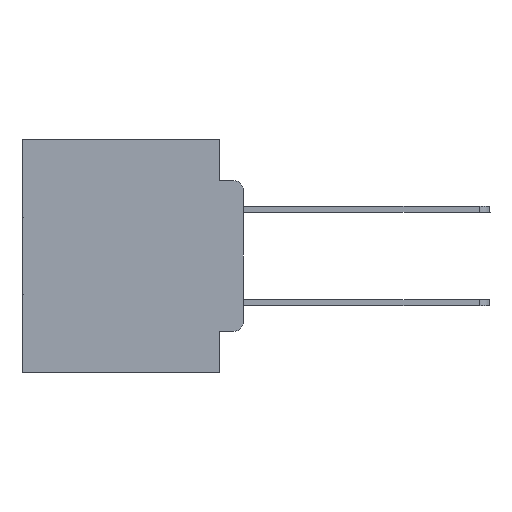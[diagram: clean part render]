
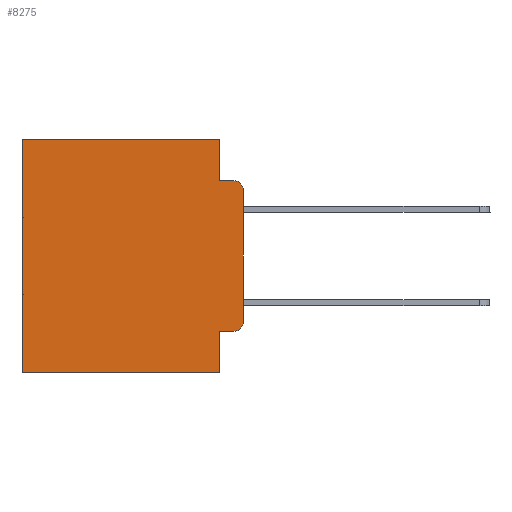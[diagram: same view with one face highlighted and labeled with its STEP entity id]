
A CAD part, left-side view. The second image highlights one B-rep face of the part: STEP entity #8275.
In plain terms, the highlighted planar face has unit normal (-1, 0, 0).
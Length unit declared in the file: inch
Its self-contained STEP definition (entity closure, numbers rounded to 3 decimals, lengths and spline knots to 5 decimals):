
#168 = EDGE_CURVE ( 'NONE', #25120, #12189, #8718, .T. ) ;
#477 = DIRECTION ( 'NONE',  ( -1., 0., 0. ) ) ;
#833 = ORIENTED_EDGE ( 'NONE', *, *, #6569, .T. ) ;
#846 = CARTESIAN_POINT ( 'NONE',  ( 0.298, 0.02, -0.1085 ) ) ;
#1362 = VERTEX_POINT ( 'NONE', #13399 ) ;
#1536 = LINE ( 'NONE', #21350, #23215 ) ;
#2084 = LINE ( 'NONE', #9286, #30839 ) ;
#3157 = VECTOR ( 'NONE', #22721, 39.37008 ) ;
#3312 = CARTESIAN_POINT ( 'NONE',  ( 0.298, 0.051, -0.4115 ) ) ;
#3322 = ORIENTED_EDGE ( 'NONE', *, *, #18138, .F. ) ;
#3607 = EDGE_CURVE ( 'NONE', #7189, #1362, #27924, .T. ) ;
#3878 = VERTEX_POINT ( 'NONE', #11503 ) ;
#6160 = CARTESIAN_POINT ( 'NONE',  ( 0.298, 0., 0. ) ) ;
#6284 = CARTESIAN_POINT ( 'NONE',  ( 0.298, 0.473, -0.5 ) ) ;
#6424 = CARTESIAN_POINT ( 'NONE',  ( 0.298, 0.02, -0.0885 ) ) ;
#6438 = ORIENTED_EDGE ( 'NONE', *, *, #168, .T. ) ;
#6569 = EDGE_CURVE ( 'NONE', #1362, #13539, #29418, .T. ) ;
#7189 = VERTEX_POINT ( 'NONE', #9818 ) ;
#7646 = EDGE_CURVE ( 'NONE', #7189, #16347, #26404, .T. ) ;
#8092 = VECTOR ( 'NONE', #24896, 39.37008 ) ;
#8214 = VECTOR ( 'NONE', #11233, 39.37008 ) ;
#8275 = ADVANCED_FACE ( 'NONE', ( #20775 ), #13402, .F. ) ;
#8387 = DIRECTION ( 'NONE',  ( 0., 0., -1. ) ) ;
#8718 = CIRCLE ( 'NONE', #17758, 0.02 ) ;
#9092 = AXIS2_PLACEMENT_3D ( 'NONE', #22032, #477, #14625 ) ;
#9286 = CARTESIAN_POINT ( 'NONE',  ( 0.298, 0.051, 0. ) ) ;
#9496 = ORIENTED_EDGE ( 'NONE', *, *, #3607, .T. ) ;
#9818 = CARTESIAN_POINT ( 'NONE',  ( 0.298, 0.051, -0.4115 ) ) ;
#10743 = CARTESIAN_POINT ( 'NONE',  ( 0.298, 0.051, 0. ) ) ;
#10947 = CARTESIAN_POINT ( 'NONE',  ( 0.298, 0.051, -0.0885 ) ) ;
#11233 = DIRECTION ( 'NONE',  ( 0., 1., 0. ) ) ;
#11503 = CARTESIAN_POINT ( 'NONE',  ( 0.298, 0.051, 0. ) ) ;
#12189 = VERTEX_POINT ( 'NONE', #6424 ) ;
#12376 = CARTESIAN_POINT ( 'NONE',  ( 0.298, 0.473, 0. ) ) ;
#12726 = DIRECTION ( 'NONE',  ( 0., 0., -1. ) ) ;
#12851 = VERTEX_POINT ( 'NONE', #6284 ) ;
#12906 = EDGE_CURVE ( 'NONE', #3878, #28937, #1536, .T. ) ;
#12908 = CARTESIAN_POINT ( 'NONE',  ( 0.298, 0., 0. ) ) ;
#13098 = DIRECTION ( 'NONE',  ( -1., 0., 0. ) ) ;
#13399 = CARTESIAN_POINT ( 'NONE',  ( 0.298, 0.02, -0.4115 ) ) ;
#13402 = PLANE ( 'NONE',  #18716 ) ;
#13539 = VERTEX_POINT ( 'NONE', #13786 ) ;
#13786 = CARTESIAN_POINT ( 'NONE',  ( 0.298, 0., -0.3915 ) ) ;
#14625 = DIRECTION ( 'NONE',  ( 0., 0., -1. ) ) ;
#14842 = VECTOR ( 'NONE', #16387, 39.37008 ) ;
#14982 = EDGE_CURVE ( 'NONE', #25120, #13539, #28704, .T. ) ;
#15454 = DIRECTION ( 'NONE',  ( 0., -1., 0. ) ) ;
#15580 = VECTOR ( 'NONE', #15454, 39.37008 ) ;
#15831 = ORIENTED_EDGE ( 'NONE', *, *, #26017, .T. ) ;
#15946 = LINE ( 'NONE', #17724, #29770 ) ;
#16347 = VERTEX_POINT ( 'NONE', #25152 ) ;
#16376 = DIRECTION ( 'NONE',  ( 0., 0., -1. ) ) ;
#16387 = DIRECTION ( 'NONE',  ( 0., 0., -1. ) ) ;
#16898 = EDGE_CURVE ( 'NONE', #28612, #12189, #17004, .T. ) ;
#17004 = LINE ( 'NONE', #10947, #3157 ) ;
#17724 = CARTESIAN_POINT ( 'NONE',  ( 0.298, 0.473, 0. ) ) ;
#17758 = AXIS2_PLACEMENT_3D ( 'NONE', #846, #13098, #8387 ) ;
#17914 = CARTESIAN_POINT ( 'NONE',  ( 0.298, 0.051, -0.0885 ) ) ;
#18138 = EDGE_CURVE ( 'NONE', #16347, #12851, #19102, .T. ) ;
#18716 = AXIS2_PLACEMENT_3D ( 'NONE', #6160, #20398, #20507 ) ;
#18958 = CARTESIAN_POINT ( 'NONE',  ( 0.298, 0., -0.1085 ) ) ;
#19037 = ORIENTED_EDGE ( 'NONE', *, *, #14982, .F. ) ;
#19102 = LINE ( 'NONE', #23244, #8214 ) ;
#20398 = DIRECTION ( 'NONE',  ( 1., 0., 0. ) ) ;
#20505 = EDGE_CURVE ( 'NONE', #3878, #28612, #2084, .T. ) ;
#20507 = DIRECTION ( 'NONE',  ( 0., 0., -1. ) ) ;
#20775 = FACE_OUTER_BOUND ( 'NONE', #28608, .T. ) ;
#21350 = CARTESIAN_POINT ( 'NONE',  ( 0.298, 0., 0. ) ) ;
#22032 = CARTESIAN_POINT ( 'NONE',  ( 0.298, 0.02, -0.3915 ) ) ;
#22721 = DIRECTION ( 'NONE',  ( 0., -1., 0. ) ) ;
#23215 = VECTOR ( 'NONE', #25855, 39.37008 ) ;
#23244 = CARTESIAN_POINT ( 'NONE',  ( 0.298, 0., -0.5 ) ) ;
#24896 = DIRECTION ( 'NONE',  ( 0., 0., -1. ) ) ;
#25120 = VERTEX_POINT ( 'NONE', #18958 ) ;
#25152 = CARTESIAN_POINT ( 'NONE',  ( 0.298, 0.051, -0.5 ) ) ;
#25855 = DIRECTION ( 'NONE',  ( 0., 1., 0. ) ) ;
#26017 = EDGE_CURVE ( 'NONE', #28937, #12851, #15946, .T. ) ;
#26404 = LINE ( 'NONE', #10743, #14842 ) ;
#27924 = LINE ( 'NONE', #3312, #15580 ) ;
#28608 = EDGE_LOOP ( 'NONE', ( #19037, #6438, #28997, #29346, #29965, #15831, #3322, #28800, #9496, #833 ) ) ;
#28612 = VERTEX_POINT ( 'NONE', #17914 ) ;
#28704 = LINE ( 'NONE', #12908, #8092 ) ;
#28800 = ORIENTED_EDGE ( 'NONE', *, *, #7646, .F. ) ;
#28937 = VERTEX_POINT ( 'NONE', #12376 ) ;
#28997 = ORIENTED_EDGE ( 'NONE', *, *, #16898, .F. ) ;
#29346 = ORIENTED_EDGE ( 'NONE', *, *, #20505, .F. ) ;
#29418 = CIRCLE ( 'NONE', #9092, 0.02 ) ;
#29770 = VECTOR ( 'NONE', #12726, 39.37008 ) ;
#29965 = ORIENTED_EDGE ( 'NONE', *, *, #12906, .T. ) ;
#30839 = VECTOR ( 'NONE', #16376, 39.37008 ) ;
